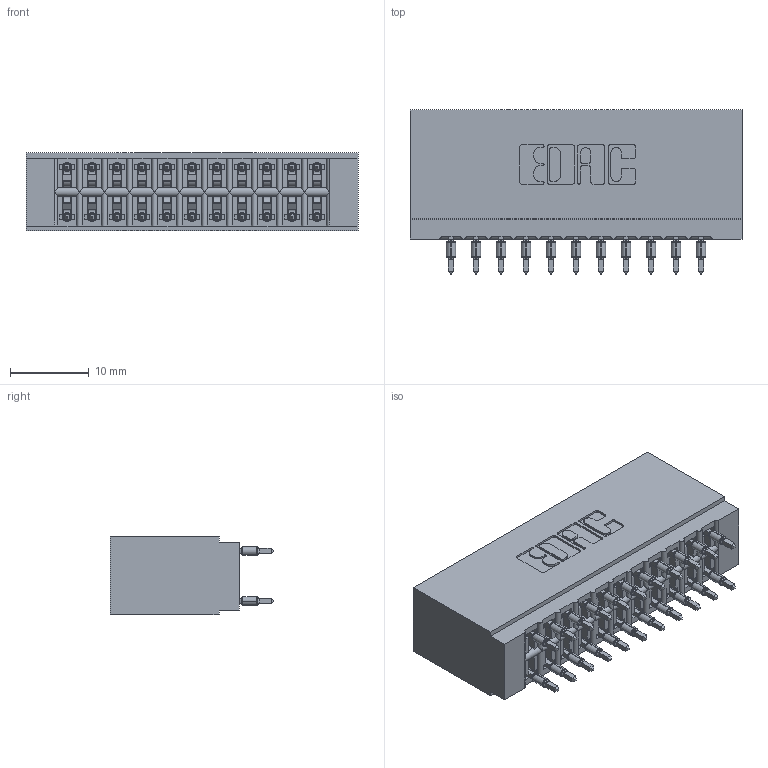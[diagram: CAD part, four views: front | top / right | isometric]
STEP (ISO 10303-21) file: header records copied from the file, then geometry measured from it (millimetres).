
FILE_DESCRIPTION (( 'STEP AP203' ), '1' );
FILE_NAME ('746-022-560-201.STEP', '2026-02-26T22:45:05', ( '' ), ( '' ), 'SwSTEP 2.0', 'SolidWorks 2023', '' );
FILE_SCHEMA (( 'CONFIG_CONTROL_DESIGN' ));
Length unit declared in the file: millimetre
Products named in the file (3): 746 Part_.515 Slot Depth - 01; 746-292-001_560; 746-022-560-201
Assembly tree (23 placements, depth 2):
  746-022-560-201
    746 Part_.515 Slot Depth - 01
    746-292-001_560  x22
Bounding box: 42.16 x 20.82 x 9.91 mm (x, y, z)
Volume: 4795.3 mm3; surface area: 7437.1 mm2
Topology: 23 solids, 23 shells, 2176 faces, 6049 edges, 3882 vertices
Faces by surface type: plane 1089, cylinder 515, bspline 440, torus 132
Entity records: 21538 total; most frequent: CARTESIAN_POINT 4549, ORIENTED_EDGE 3614, DIRECTION 3077, EDGE_CURVE 1807, VECTOR 1505, LINE 1505, VERTEX_POINT 1194, AXIS2_PLACEMENT_3D 786
